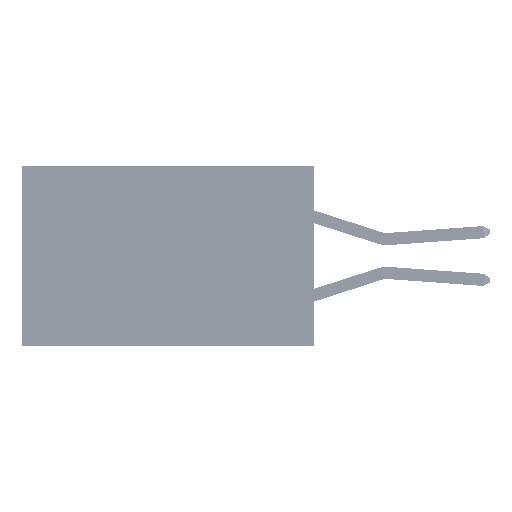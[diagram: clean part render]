
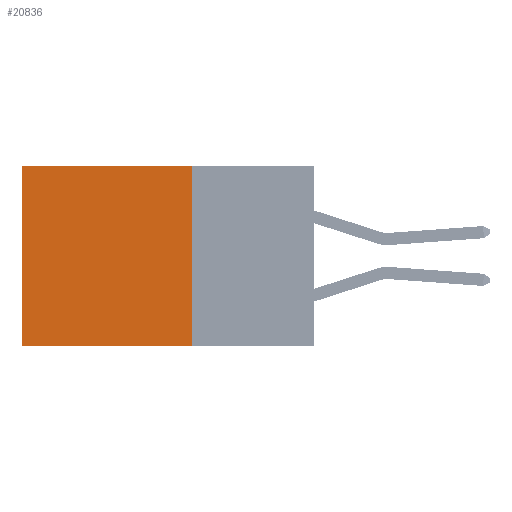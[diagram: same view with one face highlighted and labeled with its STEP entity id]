
A CAD part, left-side view. The second image highlights one B-rep face of the part: STEP entity #20836.
In plain terms, the highlighted planar face has unit normal (-1, 0, 0).
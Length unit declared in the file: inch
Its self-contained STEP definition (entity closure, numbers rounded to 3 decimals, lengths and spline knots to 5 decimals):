
#292 = CARTESIAN_POINT ( 'NONE',  ( 0.2875, 0.25, 0. ) ) ;
#2490 = CARTESIAN_POINT ( 'NONE',  ( 0.2875, 0.25, 0. ) ) ;
#2854 = ORIENTED_EDGE ( 'NONE', *, *, #7061, .T. ) ;
#3892 = VERTEX_POINT ( 'NONE', #33572 ) ;
#4844 = EDGE_CURVE ( 'NONE', #30571, #12877, #27929, .T. ) ;
#5295 = DIRECTION ( 'NONE',  ( 0., 1., 0. ) ) ;
#7061 = EDGE_CURVE ( 'NONE', #8753, #3892, #22963, .T. ) ;
#8464 = VECTOR ( 'NONE', #42070, 39.37008 ) ;
#8753 = VERTEX_POINT ( 'NONE', #32217 ) ;
#9869 = PLANE ( 'NONE',  #39145 ) ;
#12352 = DIRECTION ( 'NONE',  ( 0., 0., -1. ) ) ;
#12877 = VERTEX_POINT ( 'NONE', #33192 ) ;
#14456 = DIRECTION ( 'NONE',  ( 0., 0., -1. ) ) ;
#15350 = EDGE_LOOP ( 'NONE', ( #18189, #24244, #37910, #2854 ) ) ;
#15831 = EDGE_CURVE ( 'NONE', #8753, #30571, #32119, .T. ) ;
#15902 = VECTOR ( 'NONE', #12352, 39.37008 ) ;
#16629 = DIRECTION ( 'NONE',  ( 1., 0., 0. ) ) ;
#17329 = FACE_OUTER_BOUND ( 'NONE', #15350, .T. ) ;
#17704 = CARTESIAN_POINT ( 'NONE',  ( 0.2875, 0.25, -0.37 ) ) ;
#18189 = ORIENTED_EDGE ( 'NONE', *, *, #39483, .T. ) ;
#18451 = CARTESIAN_POINT ( 'NONE',  ( 0.2875, 0.25, -0.37 ) ) ;
#20836 = ADVANCED_FACE ( 'NONE', ( #17329 ), #9869, .F. ) ;
#22963 = LINE ( 'NONE', #2490, #25255 ) ;
#24244 = ORIENTED_EDGE ( 'NONE', *, *, #4844, .F. ) ;
#25255 = VECTOR ( 'NONE', #5295, 39.37008 ) ;
#26299 = CARTESIAN_POINT ( 'NONE',  ( 0.2875, 0.6, 0. ) ) ;
#27929 = LINE ( 'NONE', #17704, #8464 ) ;
#30571 = VERTEX_POINT ( 'NONE', #18451 ) ;
#30807 = VECTOR ( 'NONE', #14456, 39.37008 ) ;
#31027 = DIRECTION ( 'NONE',  ( 0., 0., -1. ) ) ;
#32119 = LINE ( 'NONE', #292, #30807 ) ;
#32217 = CARTESIAN_POINT ( 'NONE',  ( 0.2875, 0.25, 0. ) ) ;
#33192 = CARTESIAN_POINT ( 'NONE',  ( 0.2875, 0.6, -0.37 ) ) ;
#33572 = CARTESIAN_POINT ( 'NONE',  ( 0.2875, 0.6, 0. ) ) ;
#37910 = ORIENTED_EDGE ( 'NONE', *, *, #15831, .F. ) ;
#39145 = AXIS2_PLACEMENT_3D ( 'NONE', #41921, #16629, #31027 ) ;
#39483 = EDGE_CURVE ( 'NONE', #3892, #12877, #40220, .T. ) ;
#40220 = LINE ( 'NONE', #26299, #15902 ) ;
#41921 = CARTESIAN_POINT ( 'NONE',  ( 0.2875, 0.25, 0. ) ) ;
#42070 = DIRECTION ( 'NONE',  ( 0., 1., 0. ) ) ;
